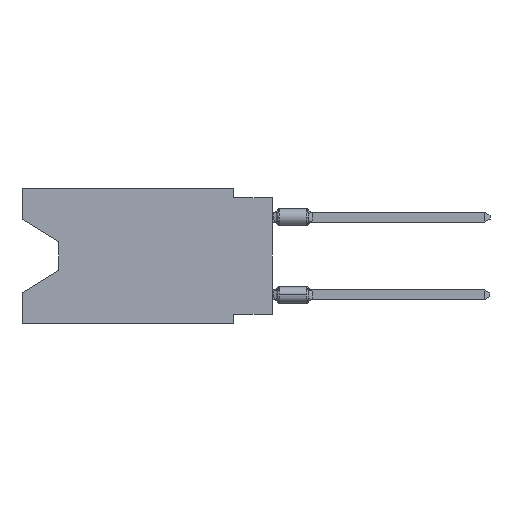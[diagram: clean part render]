
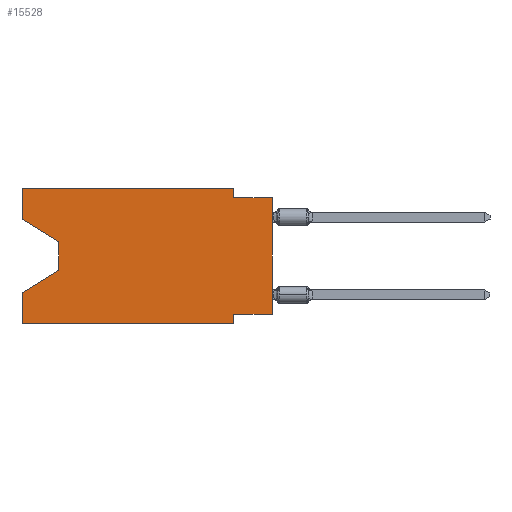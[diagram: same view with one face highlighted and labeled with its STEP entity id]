
A CAD part, left-side view. The second image highlights one B-rep face of the part: STEP entity #15528.
In plain terms, the highlighted planar face has unit normal (-1, 0, 0).
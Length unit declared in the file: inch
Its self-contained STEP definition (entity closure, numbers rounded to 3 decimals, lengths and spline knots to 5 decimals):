
#509 = LINE ( 'NONE', #16901, #35379 ) ;
#819 = EDGE_CURVE ( 'NONE', #28960, #25019, #30340, .T. ) ;
#1208 = VECTOR ( 'NONE', #25637, 39.37008 ) ;
#1708 = ORIENTED_EDGE ( 'NONE', *, *, #19272, .F. ) ;
#1776 = DIRECTION ( 'NONE',  ( 0., -1., 0. ) ) ;
#2028 = CARTESIAN_POINT ( 'NONE',  ( 0., 0.645, 0. ) ) ;
#2054 = VECTOR ( 'NONE', #1776, 39.37008 ) ;
#2287 = EDGE_CURVE ( 'NONE', #7080, #20052, #31662, .T. ) ;
#2393 = LINE ( 'NONE', #18974, #15072 ) ;
#2425 = VERTEX_POINT ( 'NONE', #6952 ) ;
#3379 = CARTESIAN_POINT ( 'NONE',  ( 0., 0.645, 0. ) ) ;
#4334 = DIRECTION ( 'NONE',  ( 0., 1., 0. ) ) ;
#4485 = VERTEX_POINT ( 'NONE', #8480 ) ;
#5854 = CARTESIAN_POINT ( 'NONE',  ( 0., 0.645, -0.35 ) ) ;
#5990 = ORIENTED_EDGE ( 'NONE', *, *, #2287, .T. ) ;
#6320 = ORIENTED_EDGE ( 'NONE', *, *, #9554, .F. ) ;
#6952 = CARTESIAN_POINT ( 'NONE',  ( 0., 0.1, -0.025 ) ) ;
#7080 = VERTEX_POINT ( 'NONE', #30488 ) ;
#7631 = ORIENTED_EDGE ( 'NONE', *, *, #36647, .F. ) ;
#7750 = VERTEX_POINT ( 'NONE', #23115 ) ;
#8014 = ORIENTED_EDGE ( 'NONE', *, *, #12004, .T. ) ;
#8310 = EDGE_CURVE ( 'NONE', #2425, #13945, #20726, .T. ) ;
#8365 = CARTESIAN_POINT ( 'NONE',  ( 0., 0.645, -0.26975 ) ) ;
#8367 = VERTEX_POINT ( 'NONE', #31129 ) ;
#8480 = CARTESIAN_POINT ( 'NONE',  ( 0., 0.1, 0. ) ) ;
#9409 = DIRECTION ( 'NONE',  ( 0., 0., 1. ) ) ;
#9554 = EDGE_CURVE ( 'NONE', #4485, #2425, #2393, .T. ) ;
#9622 = PLANE ( 'NONE',  #41756 ) ;
#10532 = CARTESIAN_POINT ( 'NONE',  ( 0., 0., -0.325 ) ) ;
#11161 = VECTOR ( 'NONE', #9409, 39.37008 ) ;
#11184 = CARTESIAN_POINT ( 'NONE',  ( 0., 0., 0. ) ) ;
#12004 = EDGE_CURVE ( 'NONE', #7750, #25019, #35031, .T. ) ;
#12664 = CARTESIAN_POINT ( 'NONE',  ( 0., 0.1, -0.35 ) ) ;
#13782 = VECTOR ( 'NONE', #17784, 39.37008 ) ;
#13945 = VERTEX_POINT ( 'NONE', #27831 ) ;
#15072 = VECTOR ( 'NONE', #19184, 39.37008 ) ;
#15265 = DIRECTION ( 'NONE',  ( 0., 0.855, -0.519 ) ) ;
#15384 = ORIENTED_EDGE ( 'NONE', *, *, #819, .F. ) ;
#15528 = ADVANCED_FACE ( 'NONE', ( #28536 ), #9622, .F. ) ;
#15561 = EDGE_CURVE ( 'NONE', #7080, #39166, #41764, .T. ) ;
#15978 = VECTOR ( 'NONE', #38868, 39.37008 ) ;
#16166 = DIRECTION ( 'NONE',  ( 0., -1., 0. ) ) ;
#16901 = CARTESIAN_POINT ( 'NONE',  ( 0., 0., -0.325 ) ) ;
#17083 = VECTOR ( 'NONE', #15265, 39.37008 ) ;
#17784 = DIRECTION ( 'NONE',  ( 0., 0., 1. ) ) ;
#17874 = CARTESIAN_POINT ( 'NONE',  ( 0., 0.645, -0.35 ) ) ;
#18239 = DIRECTION ( 'NONE',  ( 0., -1., 0. ) ) ;
#18974 = CARTESIAN_POINT ( 'NONE',  ( 0., 0.1, 0. ) ) ;
#19184 = DIRECTION ( 'NONE',  ( 0., 0., -1. ) ) ;
#19272 = EDGE_CURVE ( 'NONE', #39668, #20331, #509, .T. ) ;
#19291 = LINE ( 'NONE', #22480, #1208 ) ;
#19610 = DIRECTION ( 'NONE',  ( 0., 0., -1. ) ) ;
#20052 = VERTEX_POINT ( 'NONE', #41290 ) ;
#20331 = VERTEX_POINT ( 'NONE', #28611 ) ;
#20726 = LINE ( 'NONE', #30931, #2054 ) ;
#21333 = EDGE_CURVE ( 'NONE', #39166, #4485, #35941, .T. ) ;
#22389 = CARTESIAN_POINT ( 'NONE',  ( 0., 0.645, 0. ) ) ;
#22480 = CARTESIAN_POINT ( 'NONE',  ( 0., 0.55, -0.138 ) ) ;
#23115 = CARTESIAN_POINT ( 'NONE',  ( 0., 0.55, -0.212 ) ) ;
#23166 = EDGE_CURVE ( 'NONE', #39668, #13945, #34368, .T. ) ;
#24301 = ORIENTED_EDGE ( 'NONE', *, *, #29884, .T. ) ;
#24362 = ORIENTED_EDGE ( 'NONE', *, *, #32904, .T. ) ;
#24808 = CARTESIAN_POINT ( 'NONE',  ( 0., 0.55, -0.212 ) ) ;
#25019 = VERTEX_POINT ( 'NONE', #8365 ) ;
#25637 = DIRECTION ( 'NONE',  ( 0., 0., -1. ) ) ;
#27831 = CARTESIAN_POINT ( 'NONE',  ( 0., 0., -0.025 ) ) ;
#27969 = DIRECTION ( 'NONE',  ( 0., 0., 1. ) ) ;
#28136 = ORIENTED_EDGE ( 'NONE', *, *, #8310, .F. ) ;
#28450 = CARTESIAN_POINT ( 'NONE',  ( 0., 0.645, -0.08025 ) ) ;
#28511 = CARTESIAN_POINT ( 'NONE',  ( 0., 0.645, 0. ) ) ;
#28536 = FACE_OUTER_BOUND ( 'NONE', #33547, .T. ) ;
#28611 = CARTESIAN_POINT ( 'NONE',  ( 0., 0.1, -0.325 ) ) ;
#28896 = VECTOR ( 'NONE', #41458, 39.37008 ) ;
#28960 = VERTEX_POINT ( 'NONE', #17874 ) ;
#29884 = EDGE_CURVE ( 'NONE', #20052, #7750, #19291, .T. ) ;
#30340 = LINE ( 'NONE', #2028, #32560 ) ;
#30488 = CARTESIAN_POINT ( 'NONE',  ( 0., 0.645, -0.08025 ) ) ;
#30931 = CARTESIAN_POINT ( 'NONE',  ( 0., 0., -0.025 ) ) ;
#31129 = CARTESIAN_POINT ( 'NONE',  ( 0., 0.1, -0.35 ) ) ;
#31662 = LINE ( 'NONE', #28450, #28896 ) ;
#31959 = CARTESIAN_POINT ( 'NONE',  ( 0., 0.645, 0. ) ) ;
#32077 = ORIENTED_EDGE ( 'NONE', *, *, #21333, .F. ) ;
#32560 = VECTOR ( 'NONE', #27969, 39.37008 ) ;
#32904 = EDGE_CURVE ( 'NONE', #28960, #8367, #38024, .T. ) ;
#33547 = EDGE_LOOP ( 'NONE', ( #5990, #24301, #8014, #15384, #24362, #7631, #1708, #36208, #28136, #6320, #32077, #37923 ) ) ;
#34368 = LINE ( 'NONE', #11184, #13782 ) ;
#35031 = LINE ( 'NONE', #24808, #17083 ) ;
#35379 = VECTOR ( 'NONE', #4334, 39.37008 ) ;
#35941 = LINE ( 'NONE', #3379, #38118 ) ;
#36208 = ORIENTED_EDGE ( 'NONE', *, *, #23166, .T. ) ;
#36647 = EDGE_CURVE ( 'NONE', #20331, #8367, #41838, .T. ) ;
#37923 = ORIENTED_EDGE ( 'NONE', *, *, #15561, .F. ) ;
#38024 = LINE ( 'NONE', #5854, #40930 ) ;
#38118 = VECTOR ( 'NONE', #16166, 39.37008 ) ;
#38868 = DIRECTION ( 'NONE',  ( 0., 0., -1. ) ) ;
#39166 = VERTEX_POINT ( 'NONE', #28511 ) ;
#39668 = VERTEX_POINT ( 'NONE', #10532 ) ;
#40930 = VECTOR ( 'NONE', #18239, 39.37008 ) ;
#41290 = CARTESIAN_POINT ( 'NONE',  ( 0., 0.55, -0.138 ) ) ;
#41458 = DIRECTION ( 'NONE',  ( 0., -0.855, -0.519 ) ) ;
#41542 = DIRECTION ( 'NONE',  ( 1., 0., 0. ) ) ;
#41756 = AXIS2_PLACEMENT_3D ( 'NONE', #22389, #41542, #19610 ) ;
#41764 = LINE ( 'NONE', #31959, #11161 ) ;
#41838 = LINE ( 'NONE', #12664, #15978 ) ;
